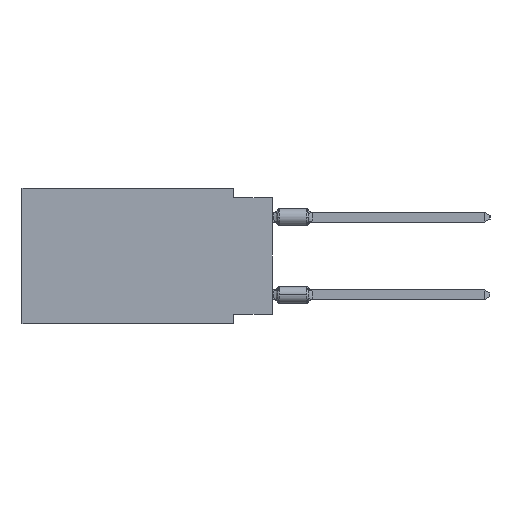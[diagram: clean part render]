
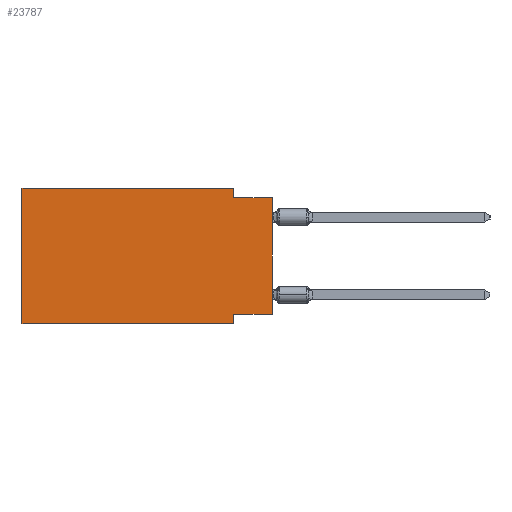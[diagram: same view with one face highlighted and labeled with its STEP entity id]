
A CAD part, left-side view. The second image highlights one B-rep face of the part: STEP entity #23787.
In plain terms, the highlighted planar face has unit normal (-1, 0, 0).
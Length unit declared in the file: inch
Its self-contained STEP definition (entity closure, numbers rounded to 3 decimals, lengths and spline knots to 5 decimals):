
#127 = EDGE_CURVE ( 'NONE', #26222, #25852, #19804, .T. ) ;
#197 = VECTOR ( 'NONE', #14372, 39.37008 ) ;
#1332 = DIRECTION ( 'NONE',  ( 0., -1., 0. ) ) ;
#1333 = CARTESIAN_POINT ( 'NONE',  ( 0., 0.1, 0. ) ) ;
#2301 = CARTESIAN_POINT ( 'NONE',  ( 0., 0.1, -0.025 ) ) ;
#3017 = VERTEX_POINT ( 'NONE', #1333 ) ;
#4805 = CARTESIAN_POINT ( 'NONE',  ( 0., 0.645, 0. ) ) ;
#5510 = VECTOR ( 'NONE', #33794, 39.37008 ) ;
#5662 = EDGE_LOOP ( 'NONE', ( #23577, #29296, #16121, #7737, #38392, #30972, #36595, #7464 ) ) ;
#5740 = EDGE_CURVE ( 'NONE', #3017, #26222, #17335, .T. ) ;
#5967 = EDGE_CURVE ( 'NONE', #31198, #25852, #9469, .T. ) ;
#6142 = LINE ( 'NONE', #18121, #31679 ) ;
#6504 = DIRECTION ( 'NONE',  ( 0., 0., 1. ) ) ;
#6734 = DIRECTION ( 'NONE',  ( 0., -1., 0. ) ) ;
#7333 = CARTESIAN_POINT ( 'NONE',  ( 0., 0., -0.325 ) ) ;
#7464 = ORIENTED_EDGE ( 'NONE', *, *, #15769, .F. ) ;
#7527 = CARTESIAN_POINT ( 'NONE',  ( 0., 0., -0.025 ) ) ;
#7737 = ORIENTED_EDGE ( 'NONE', *, *, #33292, .F. ) ;
#8536 = VERTEX_POINT ( 'NONE', #11420 ) ;
#8570 = CARTESIAN_POINT ( 'NONE',  ( 0., 0.1, -0.35 ) ) ;
#9014 = CARTESIAN_POINT ( 'NONE',  ( 0., 0.645, 0. ) ) ;
#9469 = LINE ( 'NONE', #33451, #37451 ) ;
#11222 = VECTOR ( 'NONE', #33219, 39.37008 ) ;
#11420 = CARTESIAN_POINT ( 'NONE',  ( 0., 0.1, -0.325 ) ) ;
#12986 = DIRECTION ( 'NONE',  ( 0., 0., -1. ) ) ;
#13090 = VERTEX_POINT ( 'NONE', #8570 ) ;
#13481 = EDGE_CURVE ( 'NONE', #8536, #13090, #29324, .T. ) ;
#13669 = DIRECTION ( 'NONE',  ( 0., 0., 1. ) ) ;
#14372 = DIRECTION ( 'NONE',  ( 0., 0., -1. ) ) ;
#15534 = PLANE ( 'NONE',  #21638 ) ;
#15769 = EDGE_CURVE ( 'NONE', #31198, #8536, #27704, .T. ) ;
#15808 = EDGE_CURVE ( 'NONE', #19896, #35789, #37673, .T. ) ;
#16121 = ORIENTED_EDGE ( 'NONE', *, *, #5740, .F. ) ;
#16835 = VECTOR ( 'NONE', #26771, 39.37008 ) ;
#17335 = LINE ( 'NONE', #17527, #16835 ) ;
#17527 = CARTESIAN_POINT ( 'NONE',  ( 0., 0.1, 0. ) ) ;
#18063 = LINE ( 'NONE', #9014, #11222 ) ;
#18121 = CARTESIAN_POINT ( 'NONE',  ( 0., 0.645, -0.35 ) ) ;
#18473 = FACE_OUTER_BOUND ( 'NONE', #5662, .T. ) ;
#19804 = LINE ( 'NONE', #28316, #29014 ) ;
#19896 = VERTEX_POINT ( 'NONE', #31910 ) ;
#19939 = VECTOR ( 'NONE', #13669, 39.37008 ) ;
#21638 = AXIS2_PLACEMENT_3D ( 'NONE', #27554, #30495, #12986 ) ;
#23115 = EDGE_CURVE ( 'NONE', #19896, #13090, #6142, .T. ) ;
#23577 = ORIENTED_EDGE ( 'NONE', *, *, #5967, .T. ) ;
#23787 = ADVANCED_FACE ( 'NONE', ( #18473 ), #15534, .F. ) ;
#25852 = VERTEX_POINT ( 'NONE', #7527 ) ;
#26222 = VERTEX_POINT ( 'NONE', #2301 ) ;
#26771 = DIRECTION ( 'NONE',  ( 0., 0., -1. ) ) ;
#27554 = CARTESIAN_POINT ( 'NONE',  ( 0., 0.645, 0. ) ) ;
#27704 = LINE ( 'NONE', #36730, #5510 ) ;
#28316 = CARTESIAN_POINT ( 'NONE',  ( 0., 0., -0.025 ) ) ;
#29014 = VECTOR ( 'NONE', #1332, 39.37008 ) ;
#29296 = ORIENTED_EDGE ( 'NONE', *, *, #127, .F. ) ;
#29324 = LINE ( 'NONE', #32080, #197 ) ;
#30495 = DIRECTION ( 'NONE',  ( 1., 0., 0. ) ) ;
#30972 = ORIENTED_EDGE ( 'NONE', *, *, #23115, .T. ) ;
#31198 = VERTEX_POINT ( 'NONE', #7333 ) ;
#31679 = VECTOR ( 'NONE', #6734, 39.37008 ) ;
#31910 = CARTESIAN_POINT ( 'NONE',  ( 0., 0.645, -0.35 ) ) ;
#32080 = CARTESIAN_POINT ( 'NONE',  ( 0., 0.1, -0.35 ) ) ;
#33219 = DIRECTION ( 'NONE',  ( 0., -1., 0. ) ) ;
#33292 = EDGE_CURVE ( 'NONE', #35789, #3017, #18063, .T. ) ;
#33451 = CARTESIAN_POINT ( 'NONE',  ( 0., 0., 0. ) ) ;
#33794 = DIRECTION ( 'NONE',  ( 0., 1., 0. ) ) ;
#35789 = VERTEX_POINT ( 'NONE', #37143 ) ;
#36595 = ORIENTED_EDGE ( 'NONE', *, *, #13481, .F. ) ;
#36730 = CARTESIAN_POINT ( 'NONE',  ( 0., 0., -0.325 ) ) ;
#37143 = CARTESIAN_POINT ( 'NONE',  ( 0., 0.645, 0. ) ) ;
#37451 = VECTOR ( 'NONE', #6504, 39.37008 ) ;
#37673 = LINE ( 'NONE', #4805, #19939 ) ;
#38392 = ORIENTED_EDGE ( 'NONE', *, *, #15808, .F. ) ;
